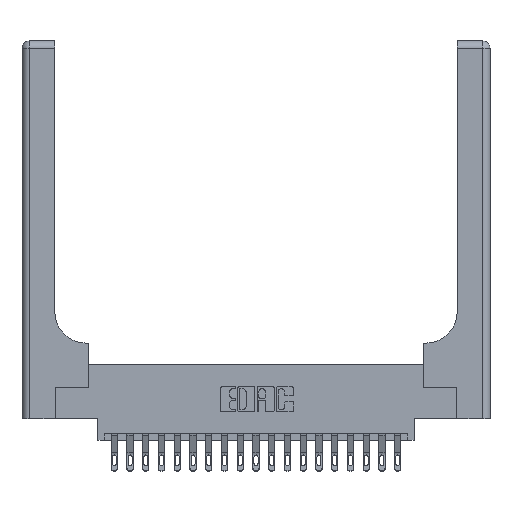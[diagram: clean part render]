
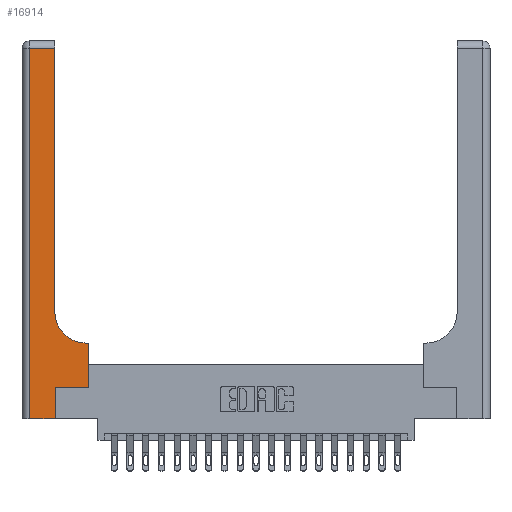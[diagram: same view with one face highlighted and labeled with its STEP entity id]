
A CAD part, top view. The second image highlights one B-rep face of the part: STEP entity #16914.
In plain terms, the highlighted planar face has unit normal (0, 0, 1).
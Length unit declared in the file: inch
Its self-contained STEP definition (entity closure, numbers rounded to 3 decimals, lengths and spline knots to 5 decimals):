
#34 = CARTESIAN_POINT ( 'NONE',  ( 0.06, 0., 0.37 ) ) ;
#148 = VERTEX_POINT ( 'NONE', #15429 ) ;
#886 = CARTESIAN_POINT ( 'NONE',  ( 0.528, 0.25, 0.37 ) ) ;
#962 = VECTOR ( 'NONE', #11667, 39.37008 ) ;
#1020 = AXIS2_PLACEMENT_3D ( 'NONE', #18363, #1644, #4917 ) ;
#1375 = CARTESIAN_POINT ( 'NONE',  ( 0.528, 0.6, 0.37 ) ) ;
#1644 = DIRECTION ( 'NONE',  ( 0., 0., -1. ) ) ;
#1720 = DIRECTION ( 'NONE',  ( 1., 0., 0. ) ) ;
#1942 = DIRECTION ( 'NONE',  ( 0., 1., 0. ) ) ;
#2047 = LINE ( 'NONE', #13974, #13962 ) ;
#2293 = CARTESIAN_POINT ( 'NONE',  ( 0.265, 0., 0.37 ) ) ;
#2552 = DIRECTION ( 'NONE',  ( 1., 0., 0. ) ) ;
#2707 = CARTESIAN_POINT ( 'NONE',  ( 0.06, 3., 0.37 ) ) ;
#2771 = EDGE_CURVE ( 'NONE', #16151, #17013, #3642, .T. ) ;
#2784 = VERTEX_POINT ( 'NONE', #10964 ) ;
#2943 = ORIENTED_EDGE ( 'NONE', *, *, #20252, .T. ) ;
#3131 = EDGE_CURVE ( 'NONE', #2784, #17642, #15871, .T. ) ;
#3315 = VERTEX_POINT ( 'NONE', #16301 ) ;
#3414 = LINE ( 'NONE', #15117, #9129 ) ;
#3642 = CIRCLE ( 'NONE', #4693, 0.25 ) ;
#4050 = DIRECTION ( 'NONE',  ( 1., 0., 0. ) ) ;
#4087 = CARTESIAN_POINT ( 'NONE',  ( 0.51, 0.85, 0.37 ) ) ;
#4298 = DIRECTION ( 'NONE',  ( 0., 0., -1. ) ) ;
#4693 = AXIS2_PLACEMENT_3D ( 'NONE', #4087, #4298, #2552 ) ;
#4888 = LINE ( 'NONE', #5103, #962 ) ;
#4917 = DIRECTION ( 'NONE',  ( -1., 0., 0. ) ) ;
#5103 = CARTESIAN_POINT ( 'NONE',  ( 0.26, 0.6, 0.37 ) ) ;
#7914 = VECTOR ( 'NONE', #19520, 39.37008 ) ;
#8457 = EDGE_CURVE ( 'NONE', #11297, #3315, #9057, .T. ) ;
#9057 = LINE ( 'NONE', #20955, #10591 ) ;
#9129 = VECTOR ( 'NONE', #16434, 39.37008 ) ;
#9494 = VECTOR ( 'NONE', #4050, 39.37008 ) ;
#9606 = VECTOR ( 'NONE', #10607, 39.37008 ) ;
#10020 = VECTOR ( 'NONE', #1720, 39.37008 ) ;
#10591 = VECTOR ( 'NONE', #10803, 39.37008 ) ;
#10607 = DIRECTION ( 'NONE',  ( 0., 1., 0. ) ) ;
#10803 = DIRECTION ( 'NONE',  ( 0., 1., 0. ) ) ;
#10964 = CARTESIAN_POINT ( 'NONE',  ( 0.528, 0.25, 0.37 ) ) ;
#11254 = ORIENTED_EDGE ( 'NONE', *, *, #3131, .T. ) ;
#11297 = VERTEX_POINT ( 'NONE', #2293 ) ;
#11648 = ORIENTED_EDGE ( 'NONE', *, *, #11706, .T. ) ;
#11667 = DIRECTION ( 'NONE',  ( -1., 0., 0. ) ) ;
#11706 = EDGE_CURVE ( 'NONE', #14037, #21266, #17570, .T. ) ;
#12501 = EDGE_LOOP ( 'NONE', ( #20241, #18738, #11648, #2943, #14061, #19403, #11254, #17734, #17225 ) ) ;
#13004 = EDGE_CURVE ( 'NONE', #17642, #16151, #4888, .T. ) ;
#13087 = EDGE_CURVE ( 'NONE', #3315, #2784, #13334, .T. ) ;
#13334 = LINE ( 'NONE', #20059, #10020 ) ;
#13962 = VECTOR ( 'NONE', #1942, 39.37008 ) ;
#13974 = CARTESIAN_POINT ( 'NONE',  ( 0.26, 3., 0.37 ) ) ;
#14037 = VERTEX_POINT ( 'NONE', #19678 ) ;
#14061 = ORIENTED_EDGE ( 'NONE', *, *, #8457, .T. ) ;
#15117 = CARTESIAN_POINT ( 'NONE',  ( 0., 2.94, 0.37 ) ) ;
#15429 = CARTESIAN_POINT ( 'NONE',  ( 0.26, 2.94, 0.37 ) ) ;
#15871 = LINE ( 'NONE', #886, #9606 ) ;
#16151 = VERTEX_POINT ( 'NONE', #19633 ) ;
#16301 = CARTESIAN_POINT ( 'NONE',  ( 0.265, 0.25, 0.37 ) ) ;
#16434 = DIRECTION ( 'NONE',  ( -1., 0., 0. ) ) ;
#16831 = PLANE ( 'NONE',  #1020 ) ;
#16914 = ADVANCED_FACE ( 'NONE', ( #19878 ), #16831, .F. ) ;
#17013 = VERTEX_POINT ( 'NONE', #17050 ) ;
#17050 = CARTESIAN_POINT ( 'NONE',  ( 0.26, 0.85, 0.37 ) ) ;
#17225 = ORIENTED_EDGE ( 'NONE', *, *, #2771, .T. ) ;
#17414 = EDGE_CURVE ( 'NONE', #17013, #148, #2047, .T. ) ;
#17570 = LINE ( 'NONE', #2707, #7914 ) ;
#17642 = VERTEX_POINT ( 'NONE', #1375 ) ;
#17734 = ORIENTED_EDGE ( 'NONE', *, *, #13004, .T. ) ;
#18363 = CARTESIAN_POINT ( 'NONE',  ( 0., 3., 0.37 ) ) ;
#18738 = ORIENTED_EDGE ( 'NONE', *, *, #19938, .T. ) ;
#19016 = LINE ( 'NONE', #19234, #9494 ) ;
#19234 = CARTESIAN_POINT ( 'NONE',  ( 0., 0., 0.37 ) ) ;
#19403 = ORIENTED_EDGE ( 'NONE', *, *, #13087, .T. ) ;
#19520 = DIRECTION ( 'NONE',  ( 0., -1., 0. ) ) ;
#19633 = CARTESIAN_POINT ( 'NONE',  ( 0.51, 0.6, 0.37 ) ) ;
#19678 = CARTESIAN_POINT ( 'NONE',  ( 0.06, 2.94, 0.37 ) ) ;
#19878 = FACE_OUTER_BOUND ( 'NONE', #12501, .T. ) ;
#19938 = EDGE_CURVE ( 'NONE', #148, #14037, #3414, .T. ) ;
#20059 = CARTESIAN_POINT ( 'NONE',  ( 0.265, 0.25, 0.37 ) ) ;
#20241 = ORIENTED_EDGE ( 'NONE', *, *, #17414, .T. ) ;
#20252 = EDGE_CURVE ( 'NONE', #21266, #11297, #19016, .T. ) ;
#20955 = CARTESIAN_POINT ( 'NONE',  ( 0.265, 0., 0.37 ) ) ;
#21266 = VERTEX_POINT ( 'NONE', #34 ) ;
